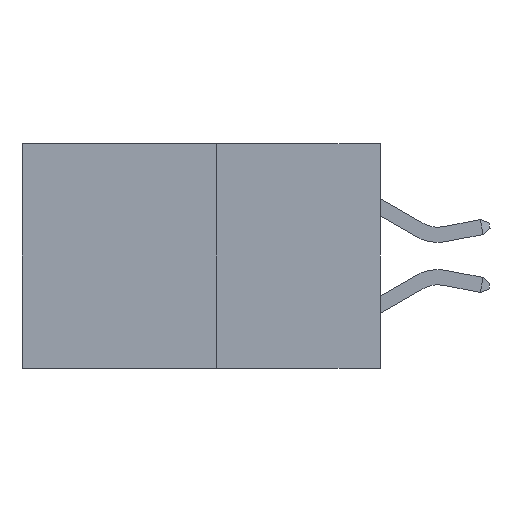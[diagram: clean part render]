
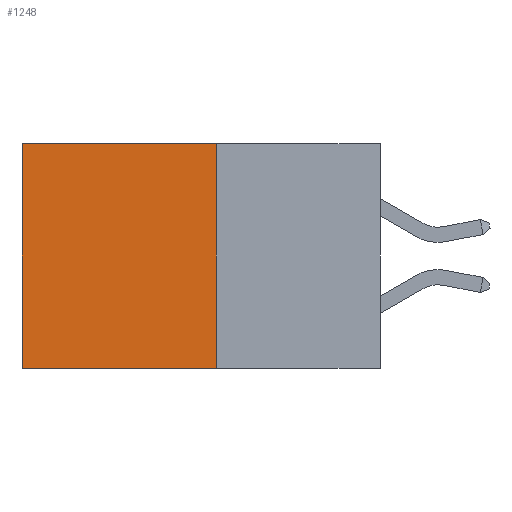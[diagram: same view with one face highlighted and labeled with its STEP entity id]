
A CAD part, left-side view. The second image highlights one B-rep face of the part: STEP entity #1248.
In plain terms, the highlighted planar face has unit normal (-1, 0, 0).
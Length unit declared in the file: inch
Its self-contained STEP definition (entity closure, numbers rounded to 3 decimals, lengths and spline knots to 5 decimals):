
#27 = EDGE_LOOP ( 'NONE', ( #2541, #11005, #7263, #10881 ) ) ;
#158 = DIRECTION ( 'NONE',  ( 0., 1., 0. ) ) ;
#852 = DIRECTION ( 'NONE',  ( 0., 1., 0. ) ) ;
#943 = EDGE_CURVE ( 'NONE', #4553, #10968, #5080, .T. ) ;
#1248 = ADVANCED_FACE ( 'NONE', ( #4710 ), #10986, .F. ) ;
#1432 = VECTOR ( 'NONE', #10007, 39.37008 ) ;
#2541 = ORIENTED_EDGE ( 'NONE', *, *, #12471, .T. ) ;
#3016 = VECTOR ( 'NONE', #12865, 39.37008 ) ;
#3740 = DIRECTION ( 'NONE',  ( 0., 0., -1. ) ) ;
#4101 = CARTESIAN_POINT ( 'NONE',  ( 0.277, 0.27, -0.37 ) ) ;
#4553 = VERTEX_POINT ( 'NONE', #9004 ) ;
#4710 = FACE_OUTER_BOUND ( 'NONE', #27, .T. ) ;
#5080 = LINE ( 'NONE', #4101, #1432 ) ;
#5154 = LINE ( 'NONE', #13059, #7634 ) ;
#5367 = CARTESIAN_POINT ( 'NONE',  ( 0.277, 0.59, -0.37 ) ) ;
#5565 = EDGE_CURVE ( 'NONE', #4553, #8508, #5154, .T. ) ;
#5959 = LINE ( 'NONE', #13855, #3016 ) ;
#6242 = AXIS2_PLACEMENT_3D ( 'NONE', #10933, #10892, #3740 ) ;
#6381 = CARTESIAN_POINT ( 'NONE',  ( 0.277, 0.27, -0.37 ) ) ;
#7263 = ORIENTED_EDGE ( 'NONE', *, *, #943, .F. ) ;
#7634 = VECTOR ( 'NONE', #158, 39.37008 ) ;
#8502 = VERTEX_POINT ( 'NONE', #5367 ) ;
#8508 = VERTEX_POINT ( 'NONE', #10616 ) ;
#9004 = CARTESIAN_POINT ( 'NONE',  ( 0.277, 0.27, 0. ) ) ;
#9204 = EDGE_CURVE ( 'NONE', #10968, #8502, #10171, .T. ) ;
#9515 = VECTOR ( 'NONE', #852, 39.37008 ) ;
#9556 = CARTESIAN_POINT ( 'NONE',  ( 0.277, 0.27, -0.37 ) ) ;
#10007 = DIRECTION ( 'NONE',  ( 0., 0., -1. ) ) ;
#10171 = LINE ( 'NONE', #9556, #9515 ) ;
#10616 = CARTESIAN_POINT ( 'NONE',  ( 0.277, 0.59, 0. ) ) ;
#10881 = ORIENTED_EDGE ( 'NONE', *, *, #5565, .T. ) ;
#10892 = DIRECTION ( 'NONE',  ( 1., 0., 0. ) ) ;
#10933 = CARTESIAN_POINT ( 'NONE',  ( 0.277, 0.27, -0.37 ) ) ;
#10968 = VERTEX_POINT ( 'NONE', #6381 ) ;
#10986 = PLANE ( 'NONE',  #6242 ) ;
#11005 = ORIENTED_EDGE ( 'NONE', *, *, #9204, .F. ) ;
#12471 = EDGE_CURVE ( 'NONE', #8508, #8502, #5959, .T. ) ;
#12865 = DIRECTION ( 'NONE',  ( 0., 0., -1. ) ) ;
#13059 = CARTESIAN_POINT ( 'NONE',  ( 0.277, 0.27, 0. ) ) ;
#13855 = CARTESIAN_POINT ( 'NONE',  ( 0.277, 0.59, -0.37 ) ) ;
